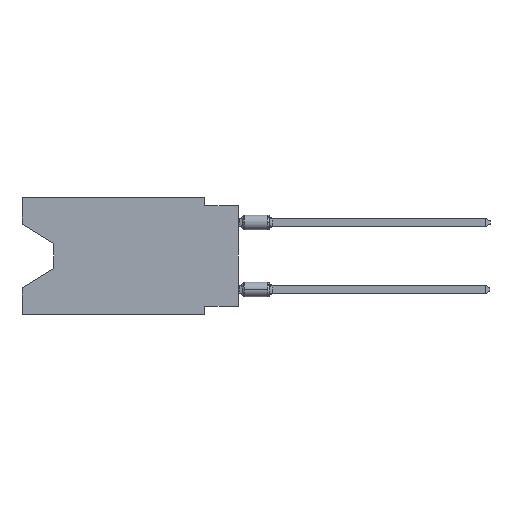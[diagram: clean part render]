
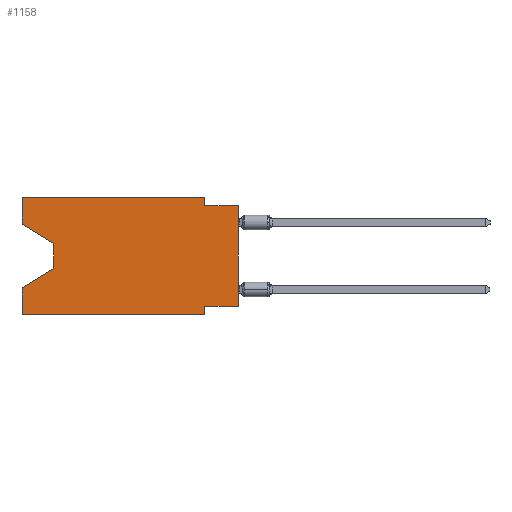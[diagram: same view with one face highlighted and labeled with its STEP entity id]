
A CAD part, left-side view. The second image highlights one B-rep face of the part: STEP entity #1158.
In plain terms, the highlighted planar face has unit normal (-1, 0, 0).
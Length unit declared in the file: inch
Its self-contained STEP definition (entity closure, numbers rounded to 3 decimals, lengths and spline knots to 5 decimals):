
#269 = DIRECTION ( 'NONE',  ( 0., 0., -1. ) ) ;
#687 = LINE ( 'NONE', #10940, #9352 ) ;
#792 = CARTESIAN_POINT ( 'NONE',  ( 0., 0.645, 0. ) ) ;
#867 = EDGE_CURVE ( 'NONE', #4097, #11417, #2308, .T. ) ;
#1104 = DIRECTION ( 'NONE',  ( 0., -1., 0. ) ) ;
#1158 = ADVANCED_FACE ( 'NONE', ( #11195 ), #8611, .F. ) ;
#1174 = CARTESIAN_POINT ( 'NONE',  ( 0., 0.1, -0.35 ) ) ;
#1350 = LINE ( 'NONE', #14045, #10898 ) ;
#1724 = VERTEX_POINT ( 'NONE', #12673 ) ;
#1785 = EDGE_CURVE ( 'NONE', #14641, #7949, #15444, .T. ) ;
#1869 = VECTOR ( 'NONE', #8698, 39.37008 ) ;
#2110 = VECTOR ( 'NONE', #2565, 39.37008 ) ;
#2308 = LINE ( 'NONE', #12560, #9879 ) ;
#2530 = ORIENTED_EDGE ( 'NONE', *, *, #11208, .F. ) ;
#2565 = DIRECTION ( 'NONE',  ( 0., 0., -1. ) ) ;
#2671 = DIRECTION ( 'NONE',  ( 0., 0., 1. ) ) ;
#2703 = DIRECTION ( 'NONE',  ( 0., 0., 1. ) ) ;
#2838 = ORIENTED_EDGE ( 'NONE', *, *, #14001, .T. ) ;
#2977 = VERTEX_POINT ( 'NONE', #4648 ) ;
#3236 = VERTEX_POINT ( 'NONE', #3509 ) ;
#3245 = DIRECTION ( 'NONE',  ( 0., -1., 0. ) ) ;
#3344 = VERTEX_POINT ( 'NONE', #4666 ) ;
#3509 = CARTESIAN_POINT ( 'NONE',  ( 0., 0., -0.325 ) ) ;
#3565 = ORIENTED_EDGE ( 'NONE', *, *, #13961, .F. ) ;
#3811 = VECTOR ( 'NONE', #4323, 39.37008 ) ;
#4026 = LINE ( 'NONE', #9054, #4341 ) ;
#4097 = VERTEX_POINT ( 'NONE', #8867 ) ;
#4323 = DIRECTION ( 'NONE',  ( 0., -0.855, -0.519 ) ) ;
#4341 = VECTOR ( 'NONE', #14027, 39.37008 ) ;
#4611 = VERTEX_POINT ( 'NONE', #15894 ) ;
#4648 = CARTESIAN_POINT ( 'NONE',  ( 0., 0.645, 0. ) ) ;
#4666 = CARTESIAN_POINT ( 'NONE',  ( 0., 0.1, -0.325 ) ) ;
#4983 = EDGE_CURVE ( 'NONE', #2977, #7767, #9711, .T. ) ;
#5050 = ORIENTED_EDGE ( 'NONE', *, *, #8937, .F. ) ;
#5068 = ORIENTED_EDGE ( 'NONE', *, *, #6531, .F. ) ;
#5296 = LINE ( 'NONE', #7896, #7187 ) ;
#5348 = VECTOR ( 'NONE', #15535, 39.37008 ) ;
#5537 = ORIENTED_EDGE ( 'NONE', *, *, #13710, .T. ) ;
#6027 = ORIENTED_EDGE ( 'NONE', *, *, #16123, .T. ) ;
#6081 = DIRECTION ( 'NONE',  ( 0., 0., -1. ) ) ;
#6257 = VERTEX_POINT ( 'NONE', #15631 ) ;
#6531 = EDGE_CURVE ( 'NONE', #7767, #15235, #16612, .T. ) ;
#6705 = EDGE_CURVE ( 'NONE', #14641, #1724, #687, .T. ) ;
#6706 = CARTESIAN_POINT ( 'NONE',  ( 0., 0.645, 0. ) ) ;
#7187 = VECTOR ( 'NONE', #13015, 39.37008 ) ;
#7335 = EDGE_CURVE ( 'NONE', #3236, #3344, #11655, .T. ) ;
#7767 = VERTEX_POINT ( 'NONE', #16343 ) ;
#7896 = CARTESIAN_POINT ( 'NONE',  ( 0., 0.645, 0. ) ) ;
#7949 = VERTEX_POINT ( 'NONE', #15579 ) ;
#8184 = CARTESIAN_POINT ( 'NONE',  ( 0., 0.645, -0.08025 ) ) ;
#8611 = PLANE ( 'NONE',  #14978 ) ;
#8698 = DIRECTION ( 'NONE',  ( 0., -1., 0. ) ) ;
#8867 = CARTESIAN_POINT ( 'NONE',  ( 0., 0.55, -0.138 ) ) ;
#8937 = EDGE_CURVE ( 'NONE', #15235, #6257, #11128, .T. ) ;
#9054 = CARTESIAN_POINT ( 'NONE',  ( 0., 0.55, -0.212 ) ) ;
#9085 = LINE ( 'NONE', #1174, #16292 ) ;
#9215 = CARTESIAN_POINT ( 'NONE',  ( 0., 0., -0.325 ) ) ;
#9352 = VECTOR ( 'NONE', #1104, 39.37008 ) ;
#9711 = LINE ( 'NONE', #13494, #11719 ) ;
#9879 = VECTOR ( 'NONE', #15178, 39.37008 ) ;
#9913 = CARTESIAN_POINT ( 'NONE',  ( 0., 0.55, -0.212 ) ) ;
#10898 = VECTOR ( 'NONE', #2703, 39.37008 ) ;
#10940 = CARTESIAN_POINT ( 'NONE',  ( 0., 0.645, -0.35 ) ) ;
#11128 = LINE ( 'NONE', #13897, #1869 ) ;
#11195 = FACE_OUTER_BOUND ( 'NONE', #12012, .T. ) ;
#11208 = EDGE_CURVE ( 'NONE', #4611, #2977, #5296, .T. ) ;
#11219 = CARTESIAN_POINT ( 'NONE',  ( 0., 0.645, -0.35 ) ) ;
#11417 = VERTEX_POINT ( 'NONE', #9913 ) ;
#11527 = ORIENTED_EDGE ( 'NONE', *, *, #4983, .F. ) ;
#11655 = LINE ( 'NONE', #9215, #5348 ) ;
#11719 = VECTOR ( 'NONE', #3245, 39.37008 ) ;
#11876 = CARTESIAN_POINT ( 'NONE',  ( 0., 0.1, -0.025 ) ) ;
#11952 = LINE ( 'NONE', #8184, #3811 ) ;
#12012 = EDGE_LOOP ( 'NONE', ( #5537, #14140, #6027, #12082, #14901, #3565, #12540, #2838, #5050, #5068, #11527, #2530 ) ) ;
#12082 = ORIENTED_EDGE ( 'NONE', *, *, #1785, .F. ) ;
#12540 = ORIENTED_EDGE ( 'NONE', *, *, #7335, .F. ) ;
#12560 = CARTESIAN_POINT ( 'NONE',  ( 0., 0.55, -0.138 ) ) ;
#12673 = CARTESIAN_POINT ( 'NONE',  ( 0., 0.1, -0.35 ) ) ;
#12909 = CARTESIAN_POINT ( 'NONE',  ( 0., 0.1, 0. ) ) ;
#13015 = DIRECTION ( 'NONE',  ( 0., 0., 1. ) ) ;
#13494 = CARTESIAN_POINT ( 'NONE',  ( 0., 0.645, 0. ) ) ;
#13710 = EDGE_CURVE ( 'NONE', #4611, #4097, #11952, .T. ) ;
#13897 = CARTESIAN_POINT ( 'NONE',  ( 0., 0., -0.025 ) ) ;
#13961 = EDGE_CURVE ( 'NONE', #3344, #1724, #9085, .T. ) ;
#14001 = EDGE_CURVE ( 'NONE', #3236, #6257, #1350, .T. ) ;
#14027 = DIRECTION ( 'NONE',  ( 0., 0.855, -0.519 ) ) ;
#14045 = CARTESIAN_POINT ( 'NONE',  ( 0., 0., 0. ) ) ;
#14140 = ORIENTED_EDGE ( 'NONE', *, *, #867, .T. ) ;
#14641 = VERTEX_POINT ( 'NONE', #11219 ) ;
#14836 = DIRECTION ( 'NONE',  ( 1., 0., 0. ) ) ;
#14901 = ORIENTED_EDGE ( 'NONE', *, *, #6705, .T. ) ;
#14978 = AXIS2_PLACEMENT_3D ( 'NONE', #792, #14836, #6081 ) ;
#15178 = DIRECTION ( 'NONE',  ( 0., 0., -1. ) ) ;
#15235 = VERTEX_POINT ( 'NONE', #11876 ) ;
#15444 = LINE ( 'NONE', #6706, #16103 ) ;
#15535 = DIRECTION ( 'NONE',  ( 0., 1., 0. ) ) ;
#15579 = CARTESIAN_POINT ( 'NONE',  ( 0., 0.645, -0.26975 ) ) ;
#15631 = CARTESIAN_POINT ( 'NONE',  ( 0., 0., -0.025 ) ) ;
#15894 = CARTESIAN_POINT ( 'NONE',  ( 0., 0.645, -0.08025 ) ) ;
#16103 = VECTOR ( 'NONE', #2671, 39.37008 ) ;
#16123 = EDGE_CURVE ( 'NONE', #11417, #7949, #4026, .T. ) ;
#16292 = VECTOR ( 'NONE', #269, 39.37008 ) ;
#16343 = CARTESIAN_POINT ( 'NONE',  ( 0., 0.1, 0. ) ) ;
#16612 = LINE ( 'NONE', #12909, #2110 ) ;
